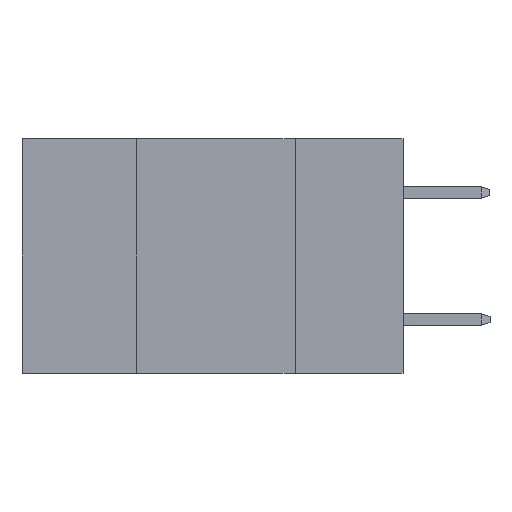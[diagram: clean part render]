
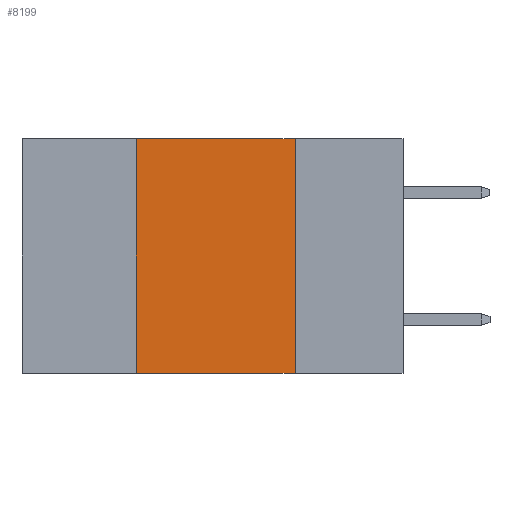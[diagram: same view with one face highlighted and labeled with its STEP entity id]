
A CAD part, left-side view. The second image highlights one B-rep face of the part: STEP entity #8199.
In plain terms, the highlighted planar face has unit normal (-1, 0, 0).
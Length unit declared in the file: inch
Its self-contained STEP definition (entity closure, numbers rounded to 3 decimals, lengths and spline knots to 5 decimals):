
#325 = VERTEX_POINT ( 'NONE', #5649 ) ;
#428 = EDGE_CURVE ( 'NONE', #2493, #325, #8839, .T. ) ;
#488 = DIRECTION ( 'NONE',  ( 0., -1., 0. ) ) ;
#1061 = DIRECTION ( 'NONE',  ( 1., 0., 0. ) ) ;
#1267 = LINE ( 'NONE', #2935, #3519 ) ;
#1464 = EDGE_CURVE ( 'NONE', #5585, #2493, #1267, .T. ) ;
#1640 = FACE_OUTER_BOUND ( 'NONE', #3422, .T. ) ;
#1951 = CARTESIAN_POINT ( 'NONE',  ( 0., 0.6, -0.37 ) ) ;
#2038 = CARTESIAN_POINT ( 'NONE',  ( 0., 0.17, 0. ) ) ;
#2139 = LINE ( 'NONE', #1951, #3322 ) ;
#2182 = DIRECTION ( 'NONE',  ( 0., -1., 0. ) ) ;
#2493 = VERTEX_POINT ( 'NONE', #2038 ) ;
#2637 = EDGE_CURVE ( 'NONE', #2825, #5585, #9751, .T. ) ;
#2825 = VERTEX_POINT ( 'NONE', #7195 ) ;
#2935 = CARTESIAN_POINT ( 'NONE',  ( 0., 0.6, 0. ) ) ;
#3262 = CARTESIAN_POINT ( 'NONE',  ( 0., 0.42, 0. ) ) ;
#3322 = VECTOR ( 'NONE', #488, 39.37008 ) ;
#3422 = EDGE_LOOP ( 'NONE', ( #8419, #7888, #7683, #4670 ) ) ;
#3494 = EDGE_CURVE ( 'NONE', #2825, #325, #2139, .T. ) ;
#3519 = VECTOR ( 'NONE', #2182, 39.37008 ) ;
#4007 = PLANE ( 'NONE',  #8546 ) ;
#4670 = ORIENTED_EDGE ( 'NONE', *, *, #3494, .T. ) ;
#4854 = CARTESIAN_POINT ( 'NONE',  ( 0., 0.6, 0. ) ) ;
#5585 = VERTEX_POINT ( 'NONE', #8912 ) ;
#5649 = CARTESIAN_POINT ( 'NONE',  ( 0., 0.17, -0.37 ) ) ;
#5845 = DIRECTION ( 'NONE',  ( 0., 0., -1. ) ) ;
#6337 = DIRECTION ( 'NONE',  ( 0., 0., 1. ) ) ;
#6553 = VECTOR ( 'NONE', #5845, 39.37008 ) ;
#6684 = VECTOR ( 'NONE', #6337, 39.37008 ) ;
#7195 = CARTESIAN_POINT ( 'NONE',  ( 0., 0.42, -0.37 ) ) ;
#7683 = ORIENTED_EDGE ( 'NONE', *, *, #2637, .F. ) ;
#7888 = ORIENTED_EDGE ( 'NONE', *, *, #1464, .F. ) ;
#8152 = CARTESIAN_POINT ( 'NONE',  ( 0., 0.17, 0. ) ) ;
#8199 = ADVANCED_FACE ( 'NONE', ( #1640 ), #4007, .F. ) ;
#8419 = ORIENTED_EDGE ( 'NONE', *, *, #428, .F. ) ;
#8546 = AXIS2_PLACEMENT_3D ( 'NONE', #4854, #1061, #8575 ) ;
#8575 = DIRECTION ( 'NONE',  ( 0., 0., -1. ) ) ;
#8839 = LINE ( 'NONE', #8152, #6553 ) ;
#8912 = CARTESIAN_POINT ( 'NONE',  ( 0., 0.42, 0. ) ) ;
#9751 = LINE ( 'NONE', #3262, #6684 ) ;
